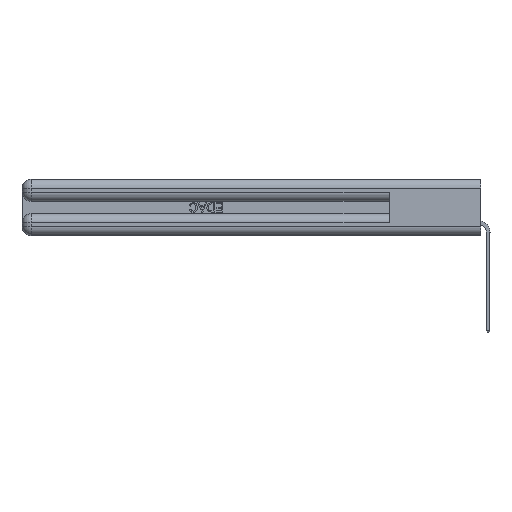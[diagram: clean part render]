
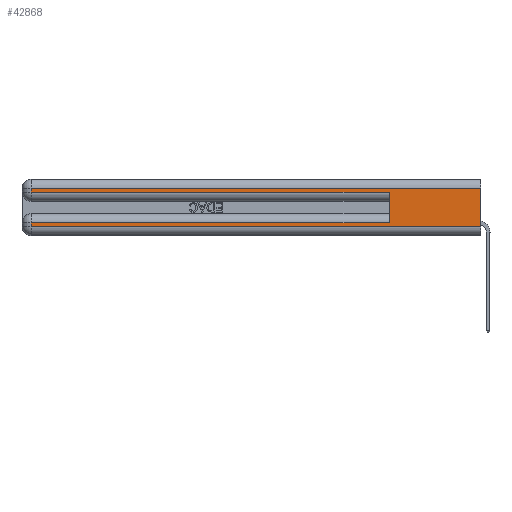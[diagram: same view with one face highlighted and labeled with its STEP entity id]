
A CAD part, left-side view. The second image highlights one B-rep face of the part: STEP entity #42868.
In plain terms, the highlighted planar face has unit normal (-1, 0, 0).
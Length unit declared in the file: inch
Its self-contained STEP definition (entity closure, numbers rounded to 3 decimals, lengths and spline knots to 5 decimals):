
#494 = LINE ( 'NONE', #44816, #12977 ) ;
#823 = FACE_OUTER_BOUND ( 'NONE', #29549, .T. ) ;
#3307 = CARTESIAN_POINT ( 'NONE',  ( 0., 0., 0.085 ) ) ;
#3353 = VECTOR ( 'NONE', #31230, 39.37008 ) ;
#5150 = LINE ( 'NONE', #3307, #38624 ) ;
#6613 = VECTOR ( 'NONE', #49306, 39.37008 ) ;
#7064 = EDGE_CURVE ( 'NONE', #36447, #22642, #42591, .T. ) ;
#8159 = EDGE_CURVE ( 'NONE', #47157, #34487, #8477, .T. ) ;
#8477 = LINE ( 'NONE', #41939, #37394 ) ;
#8592 = LINE ( 'NONE', #49837, #28313 ) ;
#8821 = DIRECTION ( 'NONE',  ( 0., 1., 0. ) ) ;
#9732 = ORIENTED_EDGE ( 'NONE', *, *, #10607, .T. ) ;
#10544 = CARTESIAN_POINT ( 'NONE',  ( 0., 0.6, 0.085 ) ) ;
#10607 = EDGE_CURVE ( 'NONE', #36448, #36447, #8592, .T. ) ;
#10927 = CARTESIAN_POINT ( 'NONE',  ( 0., 0., 0.31 ) ) ;
#11402 = CARTESIAN_POINT ( 'NONE',  ( 0., 0.6, 0.145 ) ) ;
#11803 = EDGE_CURVE ( 'NONE', #45143, #36448, #5150, .T. ) ;
#12977 = VECTOR ( 'NONE', #52356, 39.37008 ) ;
#13013 = ORIENTED_EDGE ( 'NONE', *, *, #44580, .F. ) ;
#13183 = CARTESIAN_POINT ( 'NONE',  ( 0., 0.6, 0.285 ) ) ;
#14055 = LINE ( 'NONE', #10927, #25331 ) ;
#14182 = VERTEX_POINT ( 'NONE', #36703 ) ;
#14843 = ORIENTED_EDGE ( 'NONE', *, *, #20591, .T. ) ;
#18110 = CARTESIAN_POINT ( 'NONE',  ( 0., 2.94, 0.285 ) ) ;
#20526 = DIRECTION ( 'NONE',  ( 0., 0., -1. ) ) ;
#20591 = EDGE_CURVE ( 'NONE', #38373, #14182, #14055, .T. ) ;
#21186 = PLANE ( 'NONE',  #44244 ) ;
#22586 = CARTESIAN_POINT ( 'NONE',  ( 0., 0., 0.31 ) ) ;
#22642 = VERTEX_POINT ( 'NONE', #32649 ) ;
#23107 = CARTESIAN_POINT ( 'NONE',  ( 0., 2.94, 0.06 ) ) ;
#25287 = DIRECTION ( 'NONE',  ( 0., -1., 0. ) ) ;
#25331 = VECTOR ( 'NONE', #8821, 39.37008 ) ;
#27374 = DIRECTION ( 'NONE',  ( 0., 1., 0. ) ) ;
#28313 = VECTOR ( 'NONE', #29189, 39.37008 ) ;
#29189 = DIRECTION ( 'NONE',  ( 0., 0., -1. ) ) ;
#29486 = DIRECTION ( 'NONE',  ( 1., 0., 0. ) ) ;
#29549 = EDGE_LOOP ( 'NONE', ( #42486, #14843, #37638, #42144, #13013, #41208, #9732, #47689 ) ) ;
#31019 = LINE ( 'NONE', #46516, #35596 ) ;
#31230 = DIRECTION ( 'NONE',  ( 0., -1., 0. ) ) ;
#32237 = LINE ( 'NONE', #11402, #6613 ) ;
#32649 = CARTESIAN_POINT ( 'NONE',  ( 0., 0., 0.06 ) ) ;
#33684 = EDGE_CURVE ( 'NONE', #38373, #22642, #31019, .T. ) ;
#34487 = VERTEX_POINT ( 'NONE', #13183 ) ;
#35596 = VECTOR ( 'NONE', #20526, 39.37008 ) ;
#36447 = VERTEX_POINT ( 'NONE', #23107 ) ;
#36448 = VERTEX_POINT ( 'NONE', #52540 ) ;
#36703 = CARTESIAN_POINT ( 'NONE',  ( 0., 2.94, 0.31 ) ) ;
#37394 = VECTOR ( 'NONE', #25287, 39.37008 ) ;
#37407 = DIRECTION ( 'NONE',  ( 0., 0., -1. ) ) ;
#37638 = ORIENTED_EDGE ( 'NONE', *, *, #40356, .T. ) ;
#38373 = VERTEX_POINT ( 'NONE', #22586 ) ;
#38624 = VECTOR ( 'NONE', #27374, 39.37008 ) ;
#40356 = EDGE_CURVE ( 'NONE', #14182, #47157, #494, .T. ) ;
#41208 = ORIENTED_EDGE ( 'NONE', *, *, #11803, .T. ) ;
#41939 = CARTESIAN_POINT ( 'NONE',  ( 0., 0., 0.285 ) ) ;
#42144 = ORIENTED_EDGE ( 'NONE', *, *, #8159, .T. ) ;
#42283 = CARTESIAN_POINT ( 'NONE',  ( 0., 0., 0.37 ) ) ;
#42486 = ORIENTED_EDGE ( 'NONE', *, *, #33684, .F. ) ;
#42591 = LINE ( 'NONE', #47686, #3353 ) ;
#42868 = ADVANCED_FACE ( 'NONE', ( #823 ), #21186, .F. ) ;
#44244 = AXIS2_PLACEMENT_3D ( 'NONE', #42283, #29486, #37407 ) ;
#44580 = EDGE_CURVE ( 'NONE', #45143, #34487, #32237, .T. ) ;
#44816 = CARTESIAN_POINT ( 'NONE',  ( 0., 2.94, 0.37 ) ) ;
#45143 = VERTEX_POINT ( 'NONE', #10544 ) ;
#46516 = CARTESIAN_POINT ( 'NONE',  ( 0., 0., 0.37 ) ) ;
#47157 = VERTEX_POINT ( 'NONE', #18110 ) ;
#47686 = CARTESIAN_POINT ( 'NONE',  ( 0., 0., 0.06 ) ) ;
#47689 = ORIENTED_EDGE ( 'NONE', *, *, #7064, .T. ) ;
#49306 = DIRECTION ( 'NONE',  ( 0., 0., 1. ) ) ;
#49837 = CARTESIAN_POINT ( 'NONE',  ( 0., 2.94, 0.37 ) ) ;
#52356 = DIRECTION ( 'NONE',  ( 0., 0., -1. ) ) ;
#52540 = CARTESIAN_POINT ( 'NONE',  ( 0., 2.94, 0.085 ) ) ;
